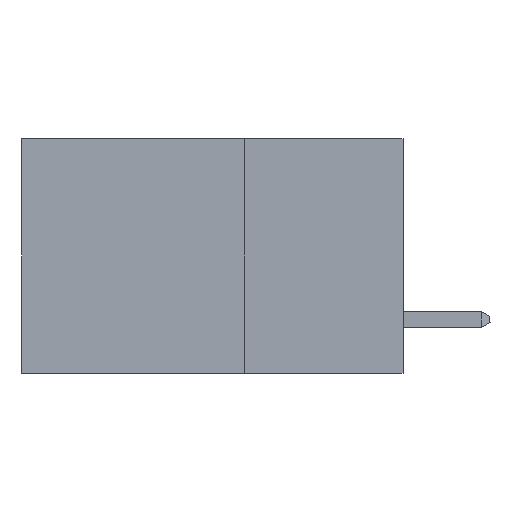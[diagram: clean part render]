
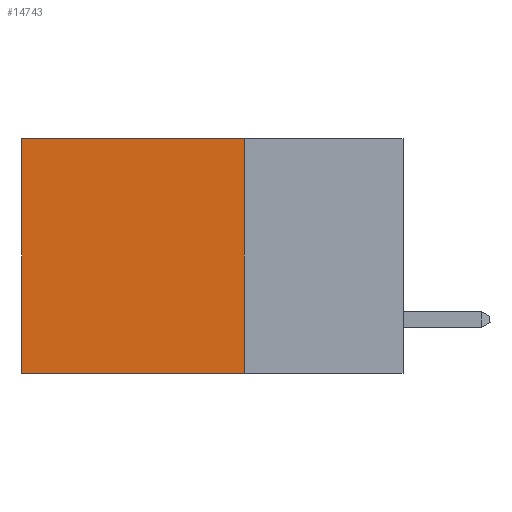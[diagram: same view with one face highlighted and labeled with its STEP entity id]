
A CAD part, left-side view. The second image highlights one B-rep face of the part: STEP entity #14743.
In plain terms, the highlighted planar face has unit normal (-1, 0, 0).
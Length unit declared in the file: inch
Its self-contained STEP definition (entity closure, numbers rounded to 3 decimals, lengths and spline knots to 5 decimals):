
#144 = DIRECTION ( 'NONE',  ( 0., 1., 0. ) ) ;
#443 = VERTEX_POINT ( 'NONE', #22965 ) ;
#869 = DIRECTION ( 'NONE',  ( 0., 0., -1. ) ) ;
#1035 = CARTESIAN_POINT ( 'NONE',  ( 0.2875, 0.25, 0. ) ) ;
#1133 = EDGE_CURVE ( 'NONE', #12735, #14208, #15221, .T. ) ;
#1318 = EDGE_LOOP ( 'NONE', ( #4964, #18285, #5244, #14411 ) ) ;
#4964 = ORIENTED_EDGE ( 'NONE', *, *, #1133, .T. ) ;
#5244 = ORIENTED_EDGE ( 'NONE', *, *, #13610, .F. ) ;
#6957 = DIRECTION ( 'NONE',  ( 0., 0., -1. ) ) ;
#7695 = VECTOR ( 'NONE', #869, 39.37008 ) ;
#8783 = LINE ( 'NONE', #18067, #15365 ) ;
#12735 = VERTEX_POINT ( 'NONE', #24038 ) ;
#12834 = CARTESIAN_POINT ( 'NONE',  ( 0.2875, 0.25, 0. ) ) ;
#12896 = CARTESIAN_POINT ( 'NONE',  ( 0.2875, 0.6, 0. ) ) ;
#13150 = DIRECTION ( 'NONE',  ( 0., 0., -1. ) ) ;
#13610 = EDGE_CURVE ( 'NONE', #23280, #443, #18756, .T. ) ;
#14208 = VERTEX_POINT ( 'NONE', #18818 ) ;
#14409 = CARTESIAN_POINT ( 'NONE',  ( 0.2875, 0.25, 0. ) ) ;
#14411 = ORIENTED_EDGE ( 'NONE', *, *, #21321, .T. ) ;
#14540 = LINE ( 'NONE', #18243, #16735 ) ;
#14650 = VECTOR ( 'NONE', #13150, 39.37008 ) ;
#14743 = ADVANCED_FACE ( 'NONE', ( #14917 ), #24796, .F. ) ;
#14917 = FACE_OUTER_BOUND ( 'NONE', #1318, .T. ) ;
#15221 = LINE ( 'NONE', #12896, #7695 ) ;
#15365 = VECTOR ( 'NONE', #144, 39.37008 ) ;
#16735 = VECTOR ( 'NONE', #22230, 39.37008 ) ;
#18067 = CARTESIAN_POINT ( 'NONE',  ( 0.2875, 0.25, 0. ) ) ;
#18243 = CARTESIAN_POINT ( 'NONE',  ( 0.2875, 0.25, -0.37 ) ) ;
#18285 = ORIENTED_EDGE ( 'NONE', *, *, #18535, .F. ) ;
#18535 = EDGE_CURVE ( 'NONE', #443, #14208, #14540, .T. ) ;
#18756 = LINE ( 'NONE', #1035, #14650 ) ;
#18818 = CARTESIAN_POINT ( 'NONE',  ( 0.2875, 0.6, -0.37 ) ) ;
#19735 = AXIS2_PLACEMENT_3D ( 'NONE', #12834, #25145, #6957 ) ;
#21321 = EDGE_CURVE ( 'NONE', #23280, #12735, #8783, .T. ) ;
#22230 = DIRECTION ( 'NONE',  ( 0., 1., 0. ) ) ;
#22965 = CARTESIAN_POINT ( 'NONE',  ( 0.2875, 0.25, -0.37 ) ) ;
#23280 = VERTEX_POINT ( 'NONE', #14409 ) ;
#24038 = CARTESIAN_POINT ( 'NONE',  ( 0.2875, 0.6, 0. ) ) ;
#24796 = PLANE ( 'NONE',  #19735 ) ;
#25145 = DIRECTION ( 'NONE',  ( 1., 0., 0. ) ) ;
